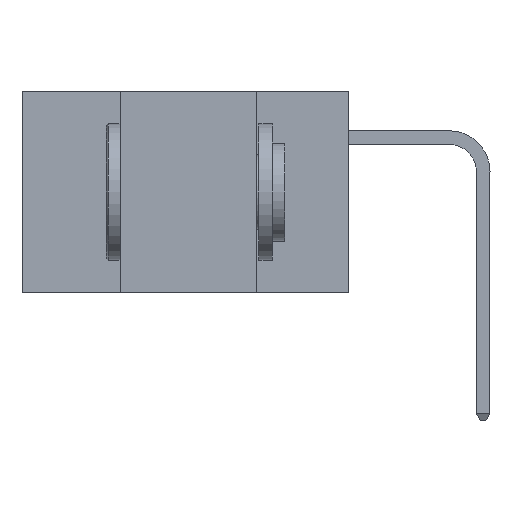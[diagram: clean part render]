
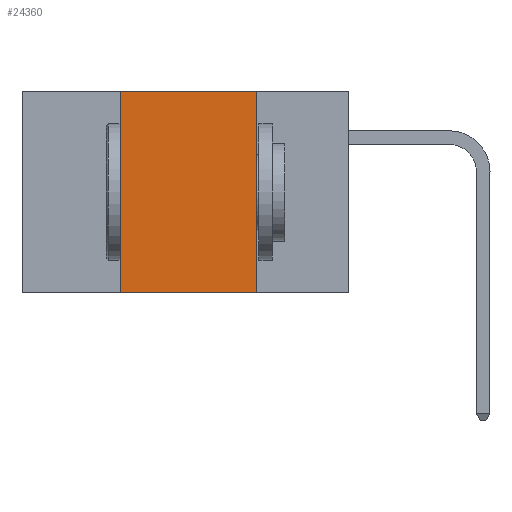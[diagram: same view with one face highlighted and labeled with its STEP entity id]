
A CAD part, left-side view. The second image highlights one B-rep face of the part: STEP entity #24360.
In plain terms, the highlighted planar face has unit normal (-1, 0, 0).
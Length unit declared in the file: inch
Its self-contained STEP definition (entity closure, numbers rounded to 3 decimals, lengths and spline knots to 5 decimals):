
#941 = EDGE_CURVE ( 'NONE', #17708, #7702, #9180, .T. ) ;
#1339 = ORIENTED_EDGE ( 'NONE', *, *, #11949, .F. ) ;
#2737 = VECTOR ( 'NONE', #11072, 39.37008 ) ;
#2940 = LINE ( 'NONE', #7842, #24337 ) ;
#3226 = EDGE_LOOP ( 'NONE', ( #1339, #21550, #23228, #16270 ) ) ;
#4130 = VECTOR ( 'NONE', #22133, 39.37008 ) ;
#4798 = CARTESIAN_POINT ( 'NONE',  ( 0., 0.6, 0. ) ) ;
#5973 = CARTESIAN_POINT ( 'NONE',  ( 0., 0.17, 0. ) ) ;
#6591 = VERTEX_POINT ( 'NONE', #5973 ) ;
#6889 = PLANE ( 'NONE',  #9985 ) ;
#7667 = CARTESIAN_POINT ( 'NONE',  ( 0., 0.17, 0. ) ) ;
#7702 = VERTEX_POINT ( 'NONE', #12556 ) ;
#7842 = CARTESIAN_POINT ( 'NONE',  ( 0., 0.42, 0. ) ) ;
#8377 = LINE ( 'NONE', #8947, #2737 ) ;
#8947 = CARTESIAN_POINT ( 'NONE',  ( 0., 0.6, 0. ) ) ;
#8975 = DIRECTION ( 'NONE',  ( 0., 0., -1. ) ) ;
#9027 = LINE ( 'NONE', #7667, #4130 ) ;
#9180 = LINE ( 'NONE', #17742, #24948 ) ;
#9985 = AXIS2_PLACEMENT_3D ( 'NONE', #4798, #15155, #8975 ) ;
#10472 = VERTEX_POINT ( 'NONE', #12942 ) ;
#11072 = DIRECTION ( 'NONE',  ( 0., -1., 0. ) ) ;
#11949 = EDGE_CURVE ( 'NONE', #6591, #7702, #9027, .T. ) ;
#12556 = CARTESIAN_POINT ( 'NONE',  ( 0., 0.17, -0.37 ) ) ;
#12942 = CARTESIAN_POINT ( 'NONE',  ( 0., 0.42, 0. ) ) ;
#14144 = DIRECTION ( 'NONE',  ( 0., 0., 1. ) ) ;
#14167 = DIRECTION ( 'NONE',  ( 0., -1., 0. ) ) ;
#14425 = EDGE_CURVE ( 'NONE', #10472, #6591, #8377, .T. ) ;
#14903 = FACE_OUTER_BOUND ( 'NONE', #3226, .T. ) ;
#15155 = DIRECTION ( 'NONE',  ( 1., 0., 0. ) ) ;
#16270 = ORIENTED_EDGE ( 'NONE', *, *, #941, .T. ) ;
#17469 = EDGE_CURVE ( 'NONE', #17708, #10472, #2940, .T. ) ;
#17708 = VERTEX_POINT ( 'NONE', #21038 ) ;
#17742 = CARTESIAN_POINT ( 'NONE',  ( 0., 0.6, -0.37 ) ) ;
#21038 = CARTESIAN_POINT ( 'NONE',  ( 0., 0.42, -0.37 ) ) ;
#21550 = ORIENTED_EDGE ( 'NONE', *, *, #14425, .F. ) ;
#22133 = DIRECTION ( 'NONE',  ( 0., 0., -1. ) ) ;
#23228 = ORIENTED_EDGE ( 'NONE', *, *, #17469, .F. ) ;
#24337 = VECTOR ( 'NONE', #14144, 39.37008 ) ;
#24360 = ADVANCED_FACE ( 'NONE', ( #14903 ), #6889, .F. ) ;
#24948 = VECTOR ( 'NONE', #14167, 39.37008 ) ;
